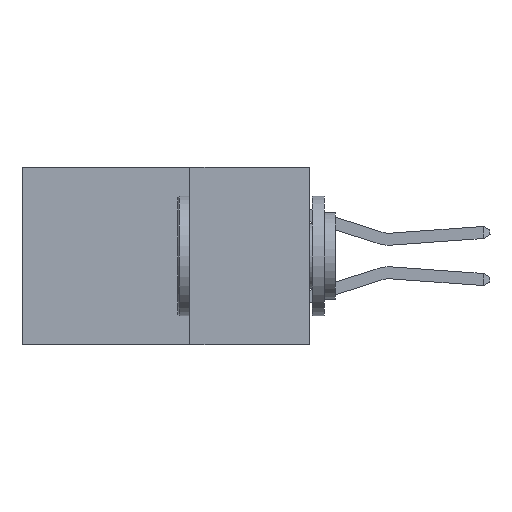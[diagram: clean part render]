
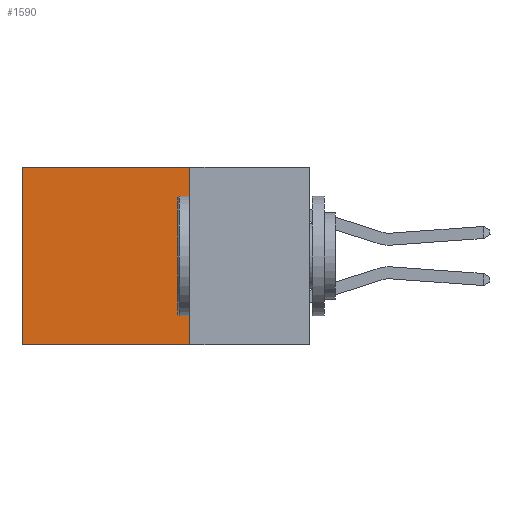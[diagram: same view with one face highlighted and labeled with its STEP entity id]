
A CAD part, left-side view. The second image highlights one B-rep face of the part: STEP entity #1590.
In plain terms, the highlighted planar face has unit normal (-1, 0, 0).
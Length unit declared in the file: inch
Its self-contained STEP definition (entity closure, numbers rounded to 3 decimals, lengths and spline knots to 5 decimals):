
#147 = CARTESIAN_POINT ( 'NONE',  ( 0.2615, 0.25, -0.37 ) ) ;
#179 = EDGE_CURVE ( 'NONE', #3470, #237, #9074, .T. ) ;
#237 = VERTEX_POINT ( 'NONE', #6201 ) ;
#438 = ORIENTED_EDGE ( 'NONE', *, *, #8327, .T. ) ;
#441 = CARTESIAN_POINT ( 'NONE',  ( 0.2615, 0.25, -0.37 ) ) ;
#470 = EDGE_CURVE ( 'NONE', #4502, #237, #3338, .T. ) ;
#1154 = VERTEX_POINT ( 'NONE', #4605 ) ;
#1284 = CARTESIAN_POINT ( 'NONE',  ( 0.2615, 0.6, -0.37 ) ) ;
#1486 = EDGE_LOOP ( 'NONE', ( #4206, #6887, #2967, #438 ) ) ;
#1590 = ADVANCED_FACE ( 'NONE', ( #7615 ), #6200, .F. ) ;
#2206 = LINE ( 'NONE', #3764, #3840 ) ;
#2579 = DIRECTION ( 'NONE',  ( 0., 1., 0. ) ) ;
#2623 = LINE ( 'NONE', #9051, #7783 ) ;
#2967 = ORIENTED_EDGE ( 'NONE', *, *, #4084, .F. ) ;
#3338 = LINE ( 'NONE', #8201, #5705 ) ;
#3470 = VERTEX_POINT ( 'NONE', #6504 ) ;
#3764 = CARTESIAN_POINT ( 'NONE',  ( 0.2615, 0.25, -0.37 ) ) ;
#3840 = VECTOR ( 'NONE', #6589, 39.37008 ) ;
#4084 = EDGE_CURVE ( 'NONE', #1154, #4502, #2206, .T. ) ;
#4206 = ORIENTED_EDGE ( 'NONE', *, *, #179, .T. ) ;
#4502 = VERTEX_POINT ( 'NONE', #147 ) ;
#4533 = VECTOR ( 'NONE', #8308, 39.37008 ) ;
#4605 = CARTESIAN_POINT ( 'NONE',  ( 0.2615, 0.25, 0. ) ) ;
#4841 = DIRECTION ( 'NONE',  ( 0., 1., 0. ) ) ;
#5705 = VECTOR ( 'NONE', #2579, 39.37008 ) ;
#6021 = DIRECTION ( 'NONE',  ( 0., 0., -1. ) ) ;
#6200 = PLANE ( 'NONE',  #8738 ) ;
#6201 = CARTESIAN_POINT ( 'NONE',  ( 0.2615, 0.6, -0.37 ) ) ;
#6504 = CARTESIAN_POINT ( 'NONE',  ( 0.2615, 0.6, 0. ) ) ;
#6589 = DIRECTION ( 'NONE',  ( 0., 0., -1. ) ) ;
#6887 = ORIENTED_EDGE ( 'NONE', *, *, #470, .F. ) ;
#7615 = FACE_OUTER_BOUND ( 'NONE', #1486, .T. ) ;
#7783 = VECTOR ( 'NONE', #4841, 39.37008 ) ;
#8201 = CARTESIAN_POINT ( 'NONE',  ( 0.2615, 0.25, -0.37 ) ) ;
#8257 = DIRECTION ( 'NONE',  ( 1., 0., 0. ) ) ;
#8308 = DIRECTION ( 'NONE',  ( 0., 0., -1. ) ) ;
#8327 = EDGE_CURVE ( 'NONE', #1154, #3470, #2623, .T. ) ;
#8738 = AXIS2_PLACEMENT_3D ( 'NONE', #441, #8257, #6021 ) ;
#9051 = CARTESIAN_POINT ( 'NONE',  ( 0.2615, 0.25, 0. ) ) ;
#9074 = LINE ( 'NONE', #1284, #4533 ) ;
